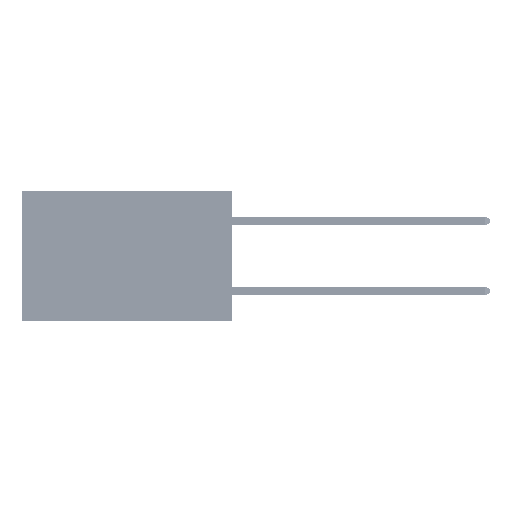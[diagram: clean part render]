
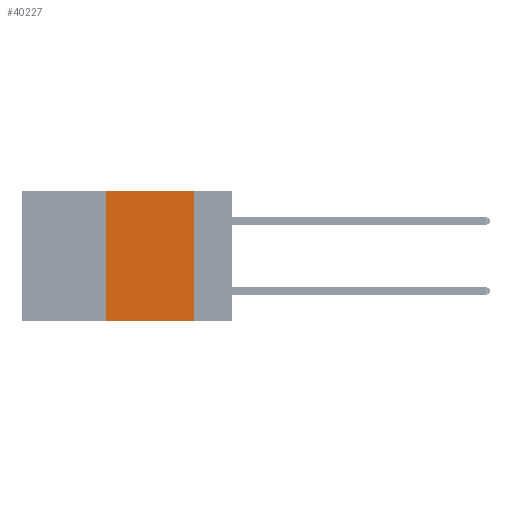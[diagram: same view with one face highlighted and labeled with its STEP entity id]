
A CAD part, left-side view. The second image highlights one B-rep face of the part: STEP entity #40227.
In plain terms, the highlighted planar face has unit normal (-1, 0, 0).
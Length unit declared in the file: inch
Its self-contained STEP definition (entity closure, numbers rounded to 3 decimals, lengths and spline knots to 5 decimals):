
#2381 = ORIENTED_EDGE ( 'NONE', *, *, #34410, .F. ) ;
#3366 = VECTOR ( 'NONE', #35775, 39.37008 ) ;
#4067 = ORIENTED_EDGE ( 'NONE', *, *, #26502, .T. ) ;
#4094 = CARTESIAN_POINT ( 'NONE',  ( 0., 0.11, 0. ) ) ;
#4136 = CARTESIAN_POINT ( 'NONE',  ( 0., 0.6, 0. ) ) ;
#4593 = DIRECTION ( 'NONE',  ( 0., 0., -1. ) ) ;
#5405 = DIRECTION ( 'NONE',  ( 0., 0., 1. ) ) ;
#5546 = ORIENTED_EDGE ( 'NONE', *, *, #27950, .F. ) ;
#10346 = FACE_OUTER_BOUND ( 'NONE', #31951, .T. ) ;
#11664 = ORIENTED_EDGE ( 'NONE', *, *, #23324, .F. ) ;
#14667 = VERTEX_POINT ( 'NONE', #24758 ) ;
#16666 = CARTESIAN_POINT ( 'NONE',  ( 0., 0.36, 0. ) ) ;
#16762 = LINE ( 'NONE', #18034, #43318 ) ;
#18034 = CARTESIAN_POINT ( 'NONE',  ( 0., 0.6, 0. ) ) ;
#19387 = DIRECTION ( 'NONE',  ( 1., 0., 0. ) ) ;
#22398 = VECTOR ( 'NONE', #4593, 39.37008 ) ;
#22585 = AXIS2_PLACEMENT_3D ( 'NONE', #4136, #19387, #31089 ) ;
#23324 = EDGE_CURVE ( 'NONE', #14667, #40844, #42059, .T. ) ;
#24249 = CARTESIAN_POINT ( 'NONE',  ( 0., 0.6, -0.37 ) ) ;
#24758 = CARTESIAN_POINT ( 'NONE',  ( 0., 0.36, -0.37 ) ) ;
#26502 = EDGE_CURVE ( 'NONE', #14667, #39846, #27453, .T. ) ;
#27453 = LINE ( 'NONE', #24249, #3366 ) ;
#27950 = EDGE_CURVE ( 'NONE', #36827, #39846, #38758, .T. ) ;
#31089 = DIRECTION ( 'NONE',  ( 0., 0., -1. ) ) ;
#31951 = EDGE_LOOP ( 'NONE', ( #5546, #2381, #11664, #4067 ) ) ;
#34410 = EDGE_CURVE ( 'NONE', #40844, #36827, #16762, .T. ) ;
#35775 = DIRECTION ( 'NONE',  ( 0., -1., 0. ) ) ;
#36368 = CARTESIAN_POINT ( 'NONE',  ( 0., 0.11, -0.37 ) ) ;
#36749 = CARTESIAN_POINT ( 'NONE',  ( 0., 0.36, 0. ) ) ;
#36827 = VERTEX_POINT ( 'NONE', #48292 ) ;
#38476 = VECTOR ( 'NONE', #5405, 39.37008 ) ;
#38758 = LINE ( 'NONE', #4094, #22398 ) ;
#39179 = PLANE ( 'NONE',  #22585 ) ;
#39846 = VERTEX_POINT ( 'NONE', #36368 ) ;
#40227 = ADVANCED_FACE ( 'NONE', ( #10346 ), #39179, .F. ) ;
#40844 = VERTEX_POINT ( 'NONE', #36749 ) ;
#42059 = LINE ( 'NONE', #16666, #38476 ) ;
#43318 = VECTOR ( 'NONE', #45372, 39.37008 ) ;
#45372 = DIRECTION ( 'NONE',  ( 0., -1., 0. ) ) ;
#48292 = CARTESIAN_POINT ( 'NONE',  ( 0., 0.11, 0. ) ) ;
